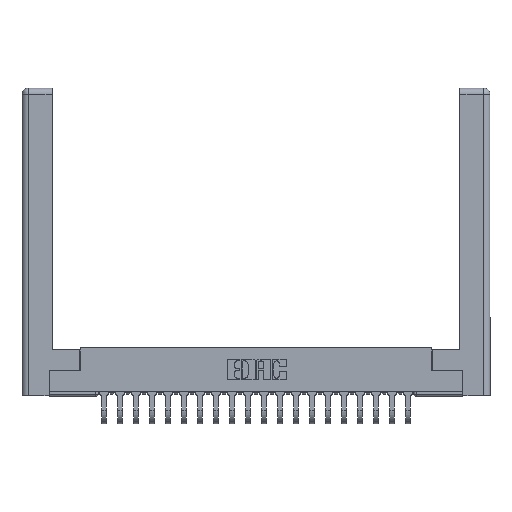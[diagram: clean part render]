
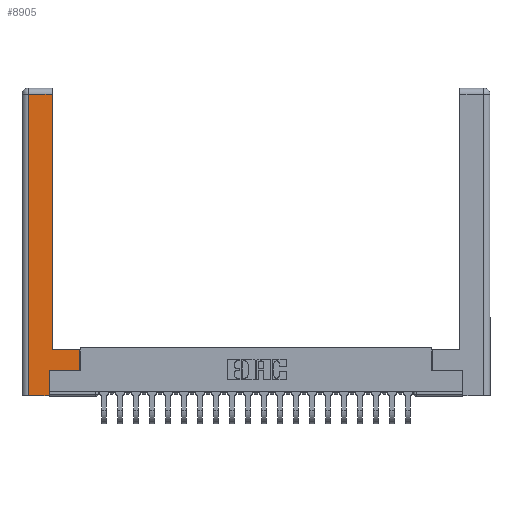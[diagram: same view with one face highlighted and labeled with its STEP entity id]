
A CAD part, top view. The second image highlights one B-rep face of the part: STEP entity #8905.
In plain terms, the highlighted planar face has unit normal (0, 0, 1).
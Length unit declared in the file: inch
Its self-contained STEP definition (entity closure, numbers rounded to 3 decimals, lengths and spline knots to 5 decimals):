
#383 = DIRECTION ( 'NONE',  ( -1., 0., 0. ) ) ;
#402 = AXIS2_PLACEMENT_3D ( 'NONE', #8870, #21097, #383 ) ;
#586 = ORIENTED_EDGE ( 'NONE', *, *, #4419, .T. ) ;
#1057 = LINE ( 'NONE', #6559, #22337 ) ;
#2103 = VERTEX_POINT ( 'NONE', #14438 ) ;
#2132 = VERTEX_POINT ( 'NONE', #7221 ) ;
#2600 = VECTOR ( 'NONE', #16782, 39.37008 ) ;
#2694 = DIRECTION ( 'NONE',  ( 0., 1., 0. ) ) ;
#3173 = ORIENTED_EDGE ( 'NONE', *, *, #9623, .T. ) ;
#3243 = DIRECTION ( 'NONE',  ( -1., 0., 0. ) ) ;
#3333 = CARTESIAN_POINT ( 'NONE',  ( 0.0615, 0., 0. ) ) ;
#3615 = CARTESIAN_POINT ( 'NONE',  ( 0.295, 3., 0. ) ) ;
#4161 = VECTOR ( 'NONE', #5488, 39.37008 ) ;
#4419 = EDGE_CURVE ( 'NONE', #20570, #15017, #12302, .T. ) ;
#4706 = LINE ( 'NONE', #21854, #12576 ) ;
#4842 = VECTOR ( 'NONE', #18651, 39.37008 ) ;
#5002 = VERTEX_POINT ( 'NONE', #14901 ) ;
#5212 = FACE_OUTER_BOUND ( 'NONE', #21815, .T. ) ;
#5488 = DIRECTION ( 'NONE',  ( 0., -1., 0. ) ) ;
#5887 = CARTESIAN_POINT ( 'NONE',  ( 0.565, 0.45, 0. ) ) ;
#6277 = VECTOR ( 'NONE', #17071, 39.37008 ) ;
#6559 = CARTESIAN_POINT ( 'NONE',  ( 0.0615, 2.94, 0. ) ) ;
#6820 = LINE ( 'NONE', #12069, #2600 ) ;
#7221 = CARTESIAN_POINT ( 'NONE',  ( 0.0615, 0., 0. ) ) ;
#7509 = ORIENTED_EDGE ( 'NONE', *, *, #12208, .T. ) ;
#7988 = ORIENTED_EDGE ( 'NONE', *, *, #17049, .T. ) ;
#8139 = CARTESIAN_POINT ( 'NONE',  ( 0.295, 0.45, 0. ) ) ;
#8769 = EDGE_CURVE ( 'NONE', #5002, #16036, #6820, .T. ) ;
#8870 = CARTESIAN_POINT ( 'NONE',  ( 0., 0., 0. ) ) ;
#8905 = ADVANCED_FACE ( 'NONE', ( #5212 ), #10696, .F. ) ;
#8936 = CARTESIAN_POINT ( 'NONE',  ( 0.265, 0., 0. ) ) ;
#9250 = EDGE_CURVE ( 'NONE', #15017, #2103, #1057, .T. ) ;
#9623 = EDGE_CURVE ( 'NONE', #16036, #20570, #14890, .T. ) ;
#9976 = DIRECTION ( 'NONE',  ( 1., 0., 0. ) ) ;
#10099 = CARTESIAN_POINT ( 'NONE',  ( 0.265, 0.245, 0. ) ) ;
#10369 = VECTOR ( 'NONE', #2694, 39.37008 ) ;
#10696 = PLANE ( 'NONE',  #402 ) ;
#11015 = EDGE_CURVE ( 'NONE', #2103, #2132, #12249, .T. ) ;
#11767 = ORIENTED_EDGE ( 'NONE', *, *, #9250, .T. ) ;
#12069 = CARTESIAN_POINT ( 'NONE',  ( 0.565, 0.45, 0. ) ) ;
#12208 = EDGE_CURVE ( 'NONE', #2132, #16726, #4706, .T. ) ;
#12249 = LINE ( 'NONE', #3333, #4161 ) ;
#12302 = LINE ( 'NONE', #3615, #10369 ) ;
#12576 = VECTOR ( 'NONE', #9976, 39.37008 ) ;
#13279 = CARTESIAN_POINT ( 'NONE',  ( 0.565, 0.245, 0. ) ) ;
#13438 = ORIENTED_EDGE ( 'NONE', *, *, #8769, .T. ) ;
#14438 = CARTESIAN_POINT ( 'NONE',  ( 0.0615, 2.94, 0. ) ) ;
#14890 = LINE ( 'NONE', #8139, #6277 ) ;
#14901 = CARTESIAN_POINT ( 'NONE',  ( 0.565, 0.245, 0. ) ) ;
#14923 = ORIENTED_EDGE ( 'NONE', *, *, #19080, .T. ) ;
#15017 = VERTEX_POINT ( 'NONE', #19132 ) ;
#15064 = DIRECTION ( 'NONE',  ( 0., 1., 0. ) ) ;
#16036 = VERTEX_POINT ( 'NONE', #5887 ) ;
#16726 = VERTEX_POINT ( 'NONE', #8936 ) ;
#16782 = DIRECTION ( 'NONE',  ( 0., 1., 0. ) ) ;
#17049 = EDGE_CURVE ( 'NONE', #21408, #5002, #21952, .T. ) ;
#17071 = DIRECTION ( 'NONE',  ( -1., 0., 0. ) ) ;
#17193 = CARTESIAN_POINT ( 'NONE',  ( 0.265, 0.245, 0. ) ) ;
#18388 = LINE ( 'NONE', #17193, #22190 ) ;
#18651 = DIRECTION ( 'NONE',  ( 1., 0., 0. ) ) ;
#19080 = EDGE_CURVE ( 'NONE', #16726, #21408, #18388, .T. ) ;
#19132 = CARTESIAN_POINT ( 'NONE',  ( 0.295, 2.94, 0. ) ) ;
#19228 = ORIENTED_EDGE ( 'NONE', *, *, #11015, .T. ) ;
#19295 = CARTESIAN_POINT ( 'NONE',  ( 0.295, 0.45, 0. ) ) ;
#20570 = VERTEX_POINT ( 'NONE', #19295 ) ;
#21097 = DIRECTION ( 'NONE',  ( 0., 0., -1. ) ) ;
#21408 = VERTEX_POINT ( 'NONE', #10099 ) ;
#21815 = EDGE_LOOP ( 'NONE', ( #586, #11767, #19228, #7509, #14923, #7988, #13438, #3173 ) ) ;
#21854 = CARTESIAN_POINT ( 'NONE',  ( 0.265, 0., 0. ) ) ;
#21952 = LINE ( 'NONE', #13279, #4842 ) ;
#22190 = VECTOR ( 'NONE', #15064, 39.37008 ) ;
#22337 = VECTOR ( 'NONE', #3243, 39.37008 ) ;
